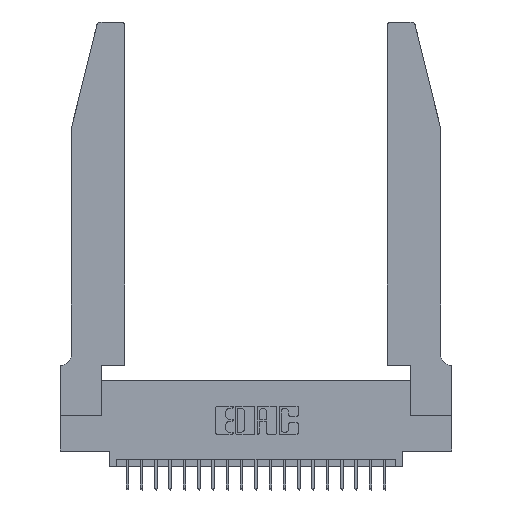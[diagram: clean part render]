
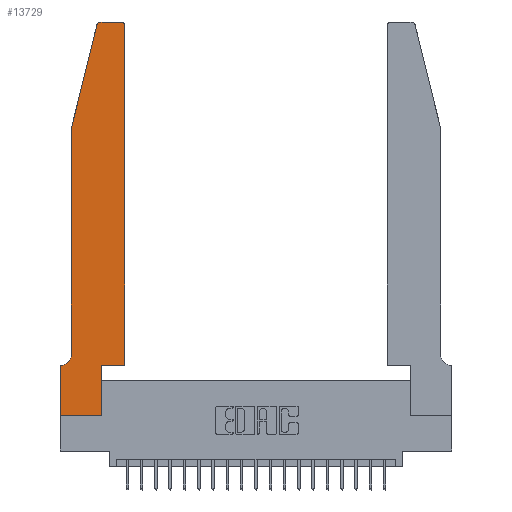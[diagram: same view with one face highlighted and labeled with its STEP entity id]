
A CAD part, top view. The second image highlights one B-rep face of the part: STEP entity #13729.
In plain terms, the highlighted planar face has unit normal (0, 0, 1).
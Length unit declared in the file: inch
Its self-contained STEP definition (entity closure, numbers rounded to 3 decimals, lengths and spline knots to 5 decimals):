
#288 = CARTESIAN_POINT ( 'NONE',  ( 0., 0., 0.37 ) ) ;
#314 = DIRECTION ( 'NONE',  ( 1., 0., 0. ) ) ;
#622 = DIRECTION ( 'NONE',  ( 1., 0., 0. ) ) ;
#660 = ORIENTED_EDGE ( 'NONE', *, *, #9631, .T. ) ;
#689 = AXIS2_PLACEMENT_3D ( 'NONE', #21851, #11534, #622 ) ;
#1076 = VERTEX_POINT ( 'NONE', #288 ) ;
#1682 = DIRECTION ( 'NONE',  ( 0., -1., 0. ) ) ;
#2300 = AXIS2_PLACEMENT_3D ( 'NONE', #10521, #22571, #12272 ) ;
#2570 = ORIENTED_EDGE ( 'NONE', *, *, #8815, .T. ) ;
#2691 = VECTOR ( 'NONE', #19995, 39.37008 ) ;
#2817 = ORIENTED_EDGE ( 'NONE', *, *, #13042, .T. ) ;
#3185 = LINE ( 'NONE', #8827, #12649 ) ;
#3680 = VERTEX_POINT ( 'NONE', #5404 ) ;
#3863 = VECTOR ( 'NONE', #14274, 39.37008 ) ;
#3904 = EDGE_CURVE ( 'NONE', #3680, #8250, #7526, .T. ) ;
#4356 = VERTEX_POINT ( 'NONE', #10819 ) ;
#4787 = CARTESIAN_POINT ( 'NONE',  ( 0.0755, 2., 0.37 ) ) ;
#5253 = VERTEX_POINT ( 'NONE', #17365 ) ;
#5404 = CARTESIAN_POINT ( 'NONE',  ( 0.4205, 2.75, 0.37 ) ) ;
#5548 = CARTESIAN_POINT ( 'NONE',  ( 0., 0.35, 0.37 ) ) ;
#5578 = ORIENTED_EDGE ( 'NONE', *, *, #9226, .T. ) ;
#6573 = DIRECTION ( 'NONE',  ( -0.239, -0.971, 0. ) ) ;
#6849 = VECTOR ( 'NONE', #6573, 39.37008 ) ;
#7044 = VECTOR ( 'NONE', #16238, 39.37008 ) ;
#7190 = VERTEX_POINT ( 'NONE', #8323 ) ;
#7375 = DIRECTION ( 'NONE',  ( 0., 0., 1. ) ) ;
#7526 = LINE ( 'NONE', #18255, #2691 ) ;
#7805 = LINE ( 'NONE', #10743, #16501 ) ;
#7845 = DIRECTION ( 'NONE',  ( -1., 0., 0. ) ) ;
#8250 = VERTEX_POINT ( 'NONE', #9449 ) ;
#8304 = VERTEX_POINT ( 'NONE', #9672 ) ;
#8323 = CARTESIAN_POINT ( 'NONE',  ( 0.0755, 0.42, 0.37 ) ) ;
#8383 = LINE ( 'NONE', #22656, #17575 ) ;
#8815 = EDGE_CURVE ( 'NONE', #13403, #7190, #19861, .T. ) ;
#8827 = CARTESIAN_POINT ( 'NONE',  ( 0.2865, 0.35, 0.37 ) ) ;
#9057 = ORIENTED_EDGE ( 'NONE', *, *, #16253, .T. ) ;
#9080 = CARTESIAN_POINT ( 'NONE',  ( 0.4505, 0.35, 0.37 ) ) ;
#9226 = EDGE_CURVE ( 'NONE', #1076, #18588, #16305, .T. ) ;
#9449 = CARTESIAN_POINT ( 'NONE',  ( 0.284, 2.75, 0.37 ) ) ;
#9592 = CARTESIAN_POINT ( 'NONE',  ( 0.2865, 0., 0.37 ) ) ;
#9631 = EDGE_CURVE ( 'NONE', #18588, #8304, #3185, .T. ) ;
#9672 = CARTESIAN_POINT ( 'NONE',  ( 0.2865, 0.35, 0.37 ) ) ;
#10044 = CARTESIAN_POINT ( 'NONE',  ( 0.0755, 2., 0.37 ) ) ;
#10086 = EDGE_CURVE ( 'NONE', #12281, #13403, #11536, .T. ) ;
#10521 = CARTESIAN_POINT ( 'NONE',  ( 0.0055, 0.42, 0.37 ) ) ;
#10564 = DIRECTION ( 'NONE',  ( 0., 1., 0. ) ) ;
#10743 = CARTESIAN_POINT ( 'NONE',  ( 0., 0., 0.37 ) ) ;
#10819 = CARTESIAN_POINT ( 'NONE',  ( 0.4505, 2.72, 0.37 ) ) ;
#11046 = CIRCLE ( 'NONE', #14260, 0.03 ) ;
#11263 = DIRECTION ( 'NONE',  ( 0., 0., 1. ) ) ;
#11359 = ORIENTED_EDGE ( 'NONE', *, *, #19287, .T. ) ;
#11534 = DIRECTION ( 'NONE',  ( 0., 0., 1. ) ) ;
#11536 = LINE ( 'NONE', #4787, #6849 ) ;
#11666 = ORIENTED_EDGE ( 'NONE', *, *, #22866, .T. ) ;
#12272 = DIRECTION ( 'NONE',  ( -1., 0., 0. ) ) ;
#12281 = VERTEX_POINT ( 'NONE', #21002 ) ;
#12351 = DIRECTION ( 'NONE',  ( 1., 0., 0. ) ) ;
#12405 = EDGE_LOOP ( 'NONE', ( #13096, #9057, #12677, #2570, #15415, #11359, #19455, #5578, #660, #11666, #2817, #19124 ) ) ;
#12445 = VERTEX_POINT ( 'NONE', #17998 ) ;
#12649 = VECTOR ( 'NONE', #10564, 39.37008 ) ;
#12677 = ORIENTED_EDGE ( 'NONE', *, *, #10086, .T. ) ;
#12783 = CARTESIAN_POINT ( 'NONE',  ( 0., 0., 0.37 ) ) ;
#13042 = EDGE_CURVE ( 'NONE', #12445, #4356, #22982, .T. ) ;
#13043 = CARTESIAN_POINT ( 'NONE',  ( 0.0755, 0.35, 0.37 ) ) ;
#13096 = ORIENTED_EDGE ( 'NONE', *, *, #3904, .T. ) ;
#13403 = VERTEX_POINT ( 'NONE', #10044 ) ;
#13729 = ADVANCED_FACE ( 'NONE', ( #16516 ), #16038, .T. ) ;
#14260 = AXIS2_PLACEMENT_3D ( 'NONE', #21583, #11263, #314 ) ;
#14274 = DIRECTION ( 'NONE',  ( 0., 1., 0. ) ) ;
#14275 = EDGE_CURVE ( 'NONE', #7190, #14567, #18904, .T. ) ;
#14441 = EDGE_CURVE ( 'NONE', #4356, #3680, #11046, .T. ) ;
#14567 = VERTEX_POINT ( 'NONE', #18591 ) ;
#14624 = DIRECTION ( 'NONE',  ( 0., -1., 0. ) ) ;
#15415 = ORIENTED_EDGE ( 'NONE', *, *, #14275, .T. ) ;
#16038 = PLANE ( 'NONE',  #18584 ) ;
#16238 = DIRECTION ( 'NONE',  ( 1., 0., 0. ) ) ;
#16253 = EDGE_CURVE ( 'NONE', #8250, #12281, #22461, .T. ) ;
#16305 = LINE ( 'NONE', #12783, #7044 ) ;
#16501 = VECTOR ( 'NONE', #1682, 39.37008 ) ;
#16516 = FACE_OUTER_BOUND ( 'NONE', #12405, .T. ) ;
#16980 = VECTOR ( 'NONE', #7845, 39.37008 ) ;
#17365 = CARTESIAN_POINT ( 'NONE',  ( 0., 0.35, 0.37 ) ) ;
#17575 = VECTOR ( 'NONE', #12351, 39.37008 ) ;
#17998 = CARTESIAN_POINT ( 'NONE',  ( 0.4505, 0.35, 0.37 ) ) ;
#18091 = CARTESIAN_POINT ( 'NONE',  ( 0.0755, 2., 0.37 ) ) ;
#18255 = CARTESIAN_POINT ( 'NONE',  ( 0.2605, 2.75, 0.37 ) ) ;
#18584 = AXIS2_PLACEMENT_3D ( 'NONE', #5548, #7375, #19537 ) ;
#18588 = VERTEX_POINT ( 'NONE', #9592 ) ;
#18591 = CARTESIAN_POINT ( 'NONE',  ( 0.0055, 0.35, 0.37 ) ) ;
#18904 = CIRCLE ( 'NONE', #2300, 0.07 ) ;
#19124 = ORIENTED_EDGE ( 'NONE', *, *, #14441, .T. ) ;
#19287 = EDGE_CURVE ( 'NONE', #14567, #5253, #22609, .T. ) ;
#19455 = ORIENTED_EDGE ( 'NONE', *, *, #22935, .T. ) ;
#19537 = DIRECTION ( 'NONE',  ( 1., 0., 0. ) ) ;
#19861 = LINE ( 'NONE', #18091, #21976 ) ;
#19995 = DIRECTION ( 'NONE',  ( -1., 0., 0. ) ) ;
#21002 = CARTESIAN_POINT ( 'NONE',  ( 0.25487, 2.72718, 0.37 ) ) ;
#21583 = CARTESIAN_POINT ( 'NONE',  ( 0.4205, 2.72, 0.37 ) ) ;
#21851 = CARTESIAN_POINT ( 'NONE',  ( 0.284, 2.72, 0.37 ) ) ;
#21976 = VECTOR ( 'NONE', #14624, 39.37008 ) ;
#22461 = CIRCLE ( 'NONE', #689, 0.03 ) ;
#22571 = DIRECTION ( 'NONE',  ( 0., 0., -1. ) ) ;
#22609 = LINE ( 'NONE', #13043, #16980 ) ;
#22656 = CARTESIAN_POINT ( 'NONE',  ( 0.4505, 0.35, 0.37 ) ) ;
#22866 = EDGE_CURVE ( 'NONE', #8304, #12445, #8383, .T. ) ;
#22935 = EDGE_CURVE ( 'NONE', #5253, #1076, #7805, .T. ) ;
#22982 = LINE ( 'NONE', #9080, #3863 ) ;
